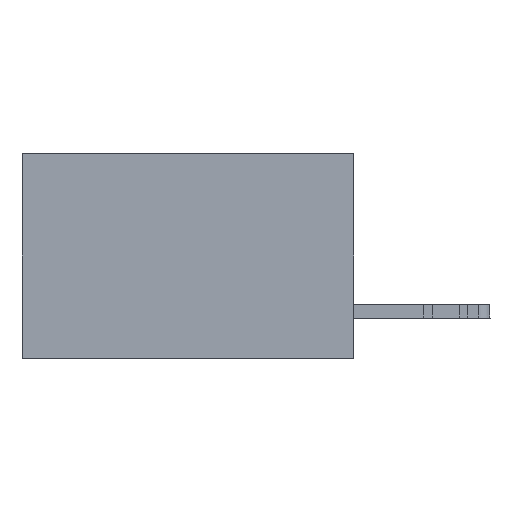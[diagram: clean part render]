
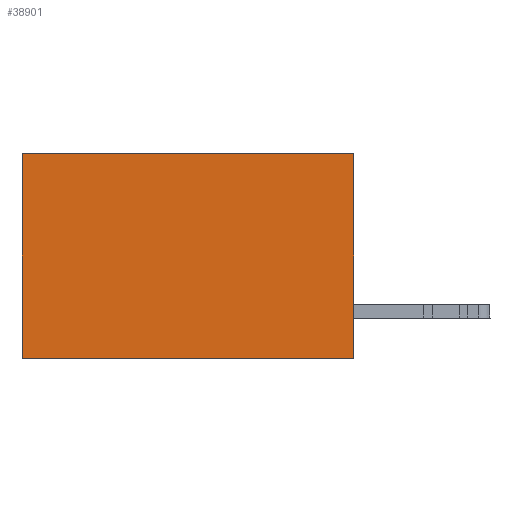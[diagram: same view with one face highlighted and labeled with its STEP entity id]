
A CAD part, left-side view. The second image highlights one B-rep face of the part: STEP entity #38901.
In plain terms, the highlighted planar face has unit normal (-1, 0, 0).
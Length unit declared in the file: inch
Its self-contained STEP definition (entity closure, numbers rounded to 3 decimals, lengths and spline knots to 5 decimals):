
#1862 = AXIS2_PLACEMENT_3D ( 'NONE', #43241, #22981, #2495 ) ;
#2495 = DIRECTION ( 'NONE',  ( 0., 0., -1. ) ) ;
#3795 = CARTESIAN_POINT ( 'NONE',  ( 0.2875, 0.6, 0. ) ) ;
#7870 = VECTOR ( 'NONE', #35750, 39.37008 ) ;
#8528 = VECTOR ( 'NONE', #17827, 39.37008 ) ;
#8675 = FACE_OUTER_BOUND ( 'NONE', #11044, .T. ) ;
#9981 = VERTEX_POINT ( 'NONE', #16347 ) ;
#10207 = LINE ( 'NONE', #39951, #30221 ) ;
#10990 = LINE ( 'NONE', #18470, #7870 ) ;
#11044 = EDGE_LOOP ( 'NONE', ( #18897, #12757, #32179, #25844 ) ) ;
#12757 = ORIENTED_EDGE ( 'NONE', *, *, #31166, .F. ) ;
#12874 = PLANE ( 'NONE',  #1862 ) ;
#13207 = CARTESIAN_POINT ( 'NONE',  ( 0.2875, 0., 0. ) ) ;
#16347 = CARTESIAN_POINT ( 'NONE',  ( 0.2875, 0., 0. ) ) ;
#17827 = DIRECTION ( 'NONE',  ( 0., 0., -1. ) ) ;
#18470 = CARTESIAN_POINT ( 'NONE',  ( 0.2875, 0., 0. ) ) ;
#18897 = ORIENTED_EDGE ( 'NONE', *, *, #26778, .T. ) ;
#18967 = EDGE_CURVE ( 'NONE', #9981, #35631, #27759, .T. ) ;
#19807 = DIRECTION ( 'NONE',  ( 0., 1., 0. ) ) ;
#20234 = CARTESIAN_POINT ( 'NONE',  ( 0.2875, 0.6, 0. ) ) ;
#20276 = DIRECTION ( 'NONE',  ( 0., 1., 0. ) ) ;
#22981 = DIRECTION ( 'NONE',  ( 1., 0., 0. ) ) ;
#23042 = VERTEX_POINT ( 'NONE', #29750 ) ;
#25844 = ORIENTED_EDGE ( 'NONE', *, *, #18967, .T. ) ;
#26778 = EDGE_CURVE ( 'NONE', #35631, #28673, #35382, .T. ) ;
#27759 = LINE ( 'NONE', #13207, #32542 ) ;
#28632 = EDGE_CURVE ( 'NONE', #9981, #23042, #10990, .T. ) ;
#28673 = VERTEX_POINT ( 'NONE', #42105 ) ;
#29750 = CARTESIAN_POINT ( 'NONE',  ( 0.2875, 0., -0.37 ) ) ;
#30221 = VECTOR ( 'NONE', #20276, 39.37008 ) ;
#31166 = EDGE_CURVE ( 'NONE', #23042, #28673, #10207, .T. ) ;
#32179 = ORIENTED_EDGE ( 'NONE', *, *, #28632, .F. ) ;
#32542 = VECTOR ( 'NONE', #19807, 39.37008 ) ;
#35382 = LINE ( 'NONE', #3795, #8528 ) ;
#35631 = VERTEX_POINT ( 'NONE', #20234 ) ;
#35750 = DIRECTION ( 'NONE',  ( 0., 0., -1. ) ) ;
#38901 = ADVANCED_FACE ( 'NONE', ( #8675 ), #12874, .F. ) ;
#39951 = CARTESIAN_POINT ( 'NONE',  ( 0.2875, 0., -0.37 ) ) ;
#42105 = CARTESIAN_POINT ( 'NONE',  ( 0.2875, 0.6, -0.37 ) ) ;
#43241 = CARTESIAN_POINT ( 'NONE',  ( 0.2875, 0., 0. ) ) ;
